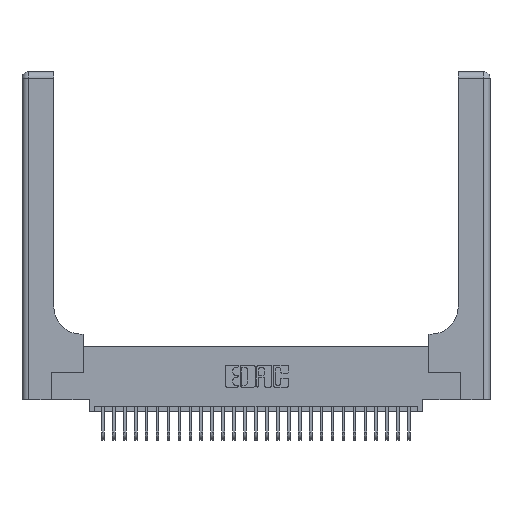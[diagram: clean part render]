
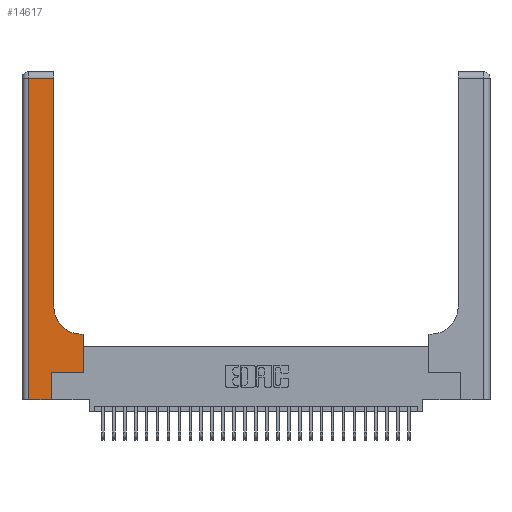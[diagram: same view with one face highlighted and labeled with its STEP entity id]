
A CAD part, top view. The second image highlights one B-rep face of the part: STEP entity #14617.
In plain terms, the highlighted planar face has unit normal (0, 0, 1).
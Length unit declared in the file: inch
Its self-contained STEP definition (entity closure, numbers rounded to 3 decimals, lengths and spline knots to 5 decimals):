
#318 = CARTESIAN_POINT ( 'NONE',  ( 0.5585, 0.25, 0.37 ) ) ;
#795 = EDGE_CURVE ( 'NONE', #10344, #12292, #11475, .T. ) ;
#1122 = EDGE_CURVE ( 'NONE', #15583, #10344, #14852, .T. ) ;
#1397 = EDGE_CURVE ( 'NONE', #6412, #11656, #14482, .T. ) ;
#1571 = VECTOR ( 'NONE', #10634, 39.37008 ) ;
#1936 = VECTOR ( 'NONE', #10599, 39.37008 ) ;
#2703 = LINE ( 'NONE', #6609, #1936 ) ;
#2835 = PLANE ( 'NONE',  #29342 ) ;
#3502 = CARTESIAN_POINT ( 'NONE',  ( 0.2915, 3., 0.37 ) ) ;
#4202 = EDGE_CURVE ( 'NONE', #9889, #10628, #24188, .T. ) ;
#4570 = CARTESIAN_POINT ( 'NONE',  ( 0., 2.94, 0.37 ) ) ;
#5227 = DIRECTION ( 'NONE',  ( 0., 1., 0. ) ) ;
#5280 = CARTESIAN_POINT ( 'NONE',  ( 0.5415, 0.6, 0.37 ) ) ;
#6412 = VERTEX_POINT ( 'NONE', #30627 ) ;
#6457 = EDGE_CURVE ( 'NONE', #23982, #6412, #2703, .T. ) ;
#6609 = CARTESIAN_POINT ( 'NONE',  ( 0.269, 0.25, 0.37 ) ) ;
#6943 = VERTEX_POINT ( 'NONE', #24835 ) ;
#7034 = LINE ( 'NONE', #11064, #15343 ) ;
#7125 = CARTESIAN_POINT ( 'NONE',  ( 0.06, 2.94, 0.37 ) ) ;
#7483 = DIRECTION ( 'NONE',  ( 1., 0., 0. ) ) ;
#7960 = DIRECTION ( 'NONE',  ( -1., 0., 0. ) ) ;
#9559 = VECTOR ( 'NONE', #5227, 39.37008 ) ;
#9679 = CARTESIAN_POINT ( 'NONE',  ( 0., 3., 0.37 ) ) ;
#9889 = VERTEX_POINT ( 'NONE', #5280 ) ;
#10022 = CARTESIAN_POINT ( 'NONE',  ( 0., 0., 0.37 ) ) ;
#10160 = EDGE_LOOP ( 'NONE', ( #20587, #17485, #28855, #29800, #30929, #14114, #25335, #19749, #31358 ) ) ;
#10260 = CARTESIAN_POINT ( 'NONE',  ( 0.269, 0.25, 0.37 ) ) ;
#10344 = VERTEX_POINT ( 'NONE', #15548 ) ;
#10599 = DIRECTION ( 'NONE',  ( 1., 0., 0. ) ) ;
#10628 = VERTEX_POINT ( 'NONE', #17568 ) ;
#10634 = DIRECTION ( 'NONE',  ( 0., 1., 0. ) ) ;
#11064 = CARTESIAN_POINT ( 'NONE',  ( 0.269, 0., 0.37 ) ) ;
#11382 = EDGE_CURVE ( 'NONE', #12292, #23982, #7034, .T. ) ;
#11475 = LINE ( 'NONE', #10022, #26321 ) ;
#11505 = DIRECTION ( 'NONE',  ( -1., 0., 0. ) ) ;
#11552 = VECTOR ( 'NONE', #21111, 39.37008 ) ;
#11656 = VERTEX_POINT ( 'NONE', #17428 ) ;
#11853 = VECTOR ( 'NONE', #11505, 39.37008 ) ;
#12292 = VERTEX_POINT ( 'NONE', #18892 ) ;
#13086 = LINE ( 'NONE', #4570, #11552 ) ;
#14114 = ORIENTED_EDGE ( 'NONE', *, *, #6457, .T. ) ;
#14482 = LINE ( 'NONE', #318, #9559 ) ;
#14552 = CARTESIAN_POINT ( 'NONE',  ( 0.5415, 0.85, 0.37 ) ) ;
#14617 = ADVANCED_FACE ( 'NONE', ( #15388 ), #2835, .F. ) ;
#14815 = EDGE_CURVE ( 'NONE', #6943, #15583, #13086, .T. ) ;
#14852 = LINE ( 'NONE', #21556, #20529 ) ;
#15343 = VECTOR ( 'NONE', #20490, 39.37008 ) ;
#15388 = FACE_OUTER_BOUND ( 'NONE', #10160, .T. ) ;
#15548 = CARTESIAN_POINT ( 'NONE',  ( 0.06, 0., 0.37 ) ) ;
#15583 = VERTEX_POINT ( 'NONE', #7125 ) ;
#17428 = CARTESIAN_POINT ( 'NONE',  ( 0.5585, 0.6, 0.37 ) ) ;
#17485 = ORIENTED_EDGE ( 'NONE', *, *, #14815, .T. ) ;
#17568 = CARTESIAN_POINT ( 'NONE',  ( 0.2915, 0.85, 0.37 ) ) ;
#18892 = CARTESIAN_POINT ( 'NONE',  ( 0.269, 0., 0.37 ) ) ;
#18893 = CARTESIAN_POINT ( 'NONE',  ( 0.2915, 0.6, 0.37 ) ) ;
#19363 = EDGE_CURVE ( 'NONE', #10628, #6943, #30909, .T. ) ;
#19394 = DIRECTION ( 'NONE',  ( 0., 0., -1. ) ) ;
#19749 = ORIENTED_EDGE ( 'NONE', *, *, #29138, .T. ) ;
#20490 = DIRECTION ( 'NONE',  ( 0., 1., 0. ) ) ;
#20529 = VECTOR ( 'NONE', #22064, 39.37008 ) ;
#20587 = ORIENTED_EDGE ( 'NONE', *, *, #19363, .T. ) ;
#21111 = DIRECTION ( 'NONE',  ( -1., 0., 0. ) ) ;
#21556 = CARTESIAN_POINT ( 'NONE',  ( 0.06, 3., 0.37 ) ) ;
#21954 = DIRECTION ( 'NONE',  ( 1., 0., 0. ) ) ;
#22064 = DIRECTION ( 'NONE',  ( 0., -1., 0. ) ) ;
#23982 = VERTEX_POINT ( 'NONE', #10260 ) ;
#24188 = CIRCLE ( 'NONE', #27173, 0.25 ) ;
#24395 = LINE ( 'NONE', #18893, #11853 ) ;
#24835 = CARTESIAN_POINT ( 'NONE',  ( 0.2915, 2.94, 0.37 ) ) ;
#25335 = ORIENTED_EDGE ( 'NONE', *, *, #1397, .T. ) ;
#26321 = VECTOR ( 'NONE', #7483, 39.37008 ) ;
#26780 = DIRECTION ( 'NONE',  ( 0., 0., -1. ) ) ;
#27173 = AXIS2_PLACEMENT_3D ( 'NONE', #14552, #26780, #21954 ) ;
#28855 = ORIENTED_EDGE ( 'NONE', *, *, #1122, .T. ) ;
#29138 = EDGE_CURVE ( 'NONE', #11656, #9889, #24395, .T. ) ;
#29342 = AXIS2_PLACEMENT_3D ( 'NONE', #9679, #19394, #7960 ) ;
#29800 = ORIENTED_EDGE ( 'NONE', *, *, #795, .T. ) ;
#30627 = CARTESIAN_POINT ( 'NONE',  ( 0.5585, 0.25, 0.37 ) ) ;
#30909 = LINE ( 'NONE', #3502, #1571 ) ;
#30929 = ORIENTED_EDGE ( 'NONE', *, *, #11382, .T. ) ;
#31358 = ORIENTED_EDGE ( 'NONE', *, *, #4202, .T. ) ;
